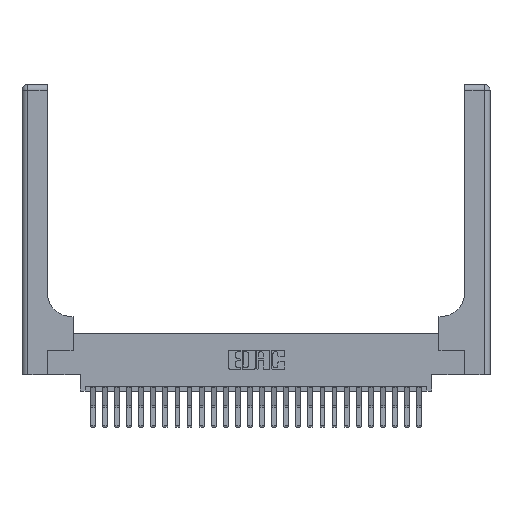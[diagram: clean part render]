
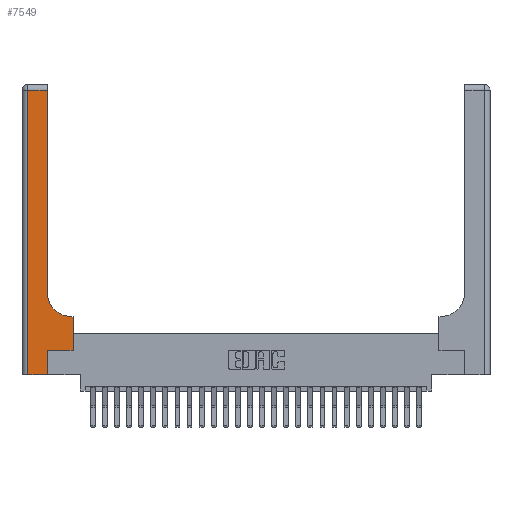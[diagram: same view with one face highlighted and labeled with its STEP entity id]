
A CAD part, top view. The second image highlights one B-rep face of the part: STEP entity #7549.
In plain terms, the highlighted planar face has unit normal (0, 0, 1).
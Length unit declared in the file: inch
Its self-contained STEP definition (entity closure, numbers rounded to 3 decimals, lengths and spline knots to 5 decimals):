
#178 = FACE_OUTER_BOUND ( 'NONE', #6360, .T. ) ;
#917 = LINE ( 'NONE', #4862, #19135 ) ;
#1280 = VECTOR ( 'NONE', #8257, 39.37008 ) ;
#1349 = VERTEX_POINT ( 'NONE', #15226 ) ;
#1555 = CARTESIAN_POINT ( 'NONE',  ( 0.528, 0.6, 0.37 ) ) ;
#2040 = EDGE_CURVE ( 'NONE', #10469, #23983, #917, .T. ) ;
#2273 = LINE ( 'NONE', #6232, #25842 ) ;
#2825 = VERTEX_POINT ( 'NONE', #14815 ) ;
#2828 = EDGE_CURVE ( 'NONE', #5490, #2825, #7042, .T. ) ;
#2840 = CARTESIAN_POINT ( 'NONE',  ( 0.265, 0., 0.37 ) ) ;
#3026 = AXIS2_PLACEMENT_3D ( 'NONE', #11907, #3858, #8357 ) ;
#3326 = LINE ( 'NONE', #9392, #13017 ) ;
#3747 = DIRECTION ( 'NONE',  ( 0., 1., 0. ) ) ;
#3858 = DIRECTION ( 'NONE',  ( 0., 0., -1. ) ) ;
#4243 = DIRECTION ( 'NONE',  ( -1., 0., 0. ) ) ;
#4377 = CARTESIAN_POINT ( 'NONE',  ( 0.26, 2.94, 0.37 ) ) ;
#4380 = CARTESIAN_POINT ( 'NONE',  ( 0.528, 0.25, 0.37 ) ) ;
#4523 = EDGE_CURVE ( 'NONE', #23983, #5490, #7577, .T. ) ;
#4862 = CARTESIAN_POINT ( 'NONE',  ( 0.265, 0.25, 0.37 ) ) ;
#5105 = EDGE_CURVE ( 'NONE', #15379, #11865, #3326, .T. ) ;
#5142 = ORIENTED_EDGE ( 'NONE', *, *, #2828, .T. ) ;
#5378 = ORIENTED_EDGE ( 'NONE', *, *, #2040, .T. ) ;
#5490 = VERTEX_POINT ( 'NONE', #1555 ) ;
#6232 = CARTESIAN_POINT ( 'NONE',  ( 0.26, 3., 0.37 ) ) ;
#6337 = VERTEX_POINT ( 'NONE', #4377 ) ;
#6360 = EDGE_LOOP ( 'NONE', ( #15680, #13267, #8103, #6695, #10920, #5378, #13872, #5142, #19883 ) ) ;
#6695 = ORIENTED_EDGE ( 'NONE', *, *, #5105, .T. ) ;
#7042 = LINE ( 'NONE', #11250, #20799 ) ;
#7549 = ADVANCED_FACE ( 'NONE', ( #178 ), #16368, .F. ) ;
#7577 = LINE ( 'NONE', #19546, #12552 ) ;
#8103 = ORIENTED_EDGE ( 'NONE', *, *, #11588, .T. ) ;
#8257 = DIRECTION ( 'NONE',  ( 0., 1., 0. ) ) ;
#8258 = CARTESIAN_POINT ( 'NONE',  ( 0.265, 0.25, 0.37 ) ) ;
#8357 = DIRECTION ( 'NONE',  ( 1., 0., 0. ) ) ;
#8659 = VECTOR ( 'NONE', #4243, 39.37008 ) ;
#8679 = VECTOR ( 'NONE', #23426, 39.37008 ) ;
#9171 = VERTEX_POINT ( 'NONE', #10102 ) ;
#9224 = CARTESIAN_POINT ( 'NONE',  ( 0.06, 3., 0.37 ) ) ;
#9392 = CARTESIAN_POINT ( 'NONE',  ( 0., 0., 0.37 ) ) ;
#9555 = EDGE_CURVE ( 'NONE', #2825, #9171, #21939, .T. ) ;
#10102 = CARTESIAN_POINT ( 'NONE',  ( 0.26, 0.85, 0.37 ) ) ;
#10469 = VERTEX_POINT ( 'NONE', #8258 ) ;
#10623 = CARTESIAN_POINT ( 'NONE',  ( 0.265, 0., 0.37 ) ) ;
#10920 = ORIENTED_EDGE ( 'NONE', *, *, #25569, .T. ) ;
#11250 = CARTESIAN_POINT ( 'NONE',  ( 0.26, 0.6, 0.37 ) ) ;
#11588 = EDGE_CURVE ( 'NONE', #1349, #15379, #21054, .T. ) ;
#11865 = VERTEX_POINT ( 'NONE', #2840 ) ;
#11907 = CARTESIAN_POINT ( 'NONE',  ( 0.51, 0.85, 0.37 ) ) ;
#12552 = VECTOR ( 'NONE', #3747, 39.37008 ) ;
#12703 = CARTESIAN_POINT ( 'NONE',  ( 0., 3., 0.37 ) ) ;
#13017 = VECTOR ( 'NONE', #15447, 39.37008 ) ;
#13267 = ORIENTED_EDGE ( 'NONE', *, *, #17519, .T. ) ;
#13872 = ORIENTED_EDGE ( 'NONE', *, *, #4523, .T. ) ;
#14219 = EDGE_CURVE ( 'NONE', #9171, #6337, #2273, .T. ) ;
#14281 = DIRECTION ( 'NONE',  ( 0., 1., 0. ) ) ;
#14815 = CARTESIAN_POINT ( 'NONE',  ( 0.51, 0.6, 0.37 ) ) ;
#15226 = CARTESIAN_POINT ( 'NONE',  ( 0.06, 2.94, 0.37 ) ) ;
#15379 = VERTEX_POINT ( 'NONE', #22969 ) ;
#15447 = DIRECTION ( 'NONE',  ( 1., 0., 0. ) ) ;
#15680 = ORIENTED_EDGE ( 'NONE', *, *, #14219, .T. ) ;
#16036 = AXIS2_PLACEMENT_3D ( 'NONE', #12703, #20169, #20302 ) ;
#16360 = CARTESIAN_POINT ( 'NONE',  ( 0., 2.94, 0.37 ) ) ;
#16368 = PLANE ( 'NONE',  #16036 ) ;
#16789 = DIRECTION ( 'NONE',  ( -1., 0., 0. ) ) ;
#17519 = EDGE_CURVE ( 'NONE', #6337, #1349, #22271, .T. ) ;
#19135 = VECTOR ( 'NONE', #22902, 39.37008 ) ;
#19546 = CARTESIAN_POINT ( 'NONE',  ( 0.528, 0.25, 0.37 ) ) ;
#19883 = ORIENTED_EDGE ( 'NONE', *, *, #9555, .T. ) ;
#20169 = DIRECTION ( 'NONE',  ( 0., 0., -1. ) ) ;
#20302 = DIRECTION ( 'NONE',  ( -1., 0., 0. ) ) ;
#20799 = VECTOR ( 'NONE', #16789, 39.37008 ) ;
#21054 = LINE ( 'NONE', #9224, #8679 ) ;
#21939 = CIRCLE ( 'NONE', #3026, 0.25 ) ;
#22271 = LINE ( 'NONE', #16360, #8659 ) ;
#22902 = DIRECTION ( 'NONE',  ( 1., 0., 0. ) ) ;
#22969 = CARTESIAN_POINT ( 'NONE',  ( 0.06, 0., 0.37 ) ) ;
#23426 = DIRECTION ( 'NONE',  ( 0., -1., 0. ) ) ;
#23983 = VERTEX_POINT ( 'NONE', #4380 ) ;
#24565 = LINE ( 'NONE', #10623, #1280 ) ;
#25569 = EDGE_CURVE ( 'NONE', #11865, #10469, #24565, .T. ) ;
#25842 = VECTOR ( 'NONE', #14281, 39.37008 ) ;
